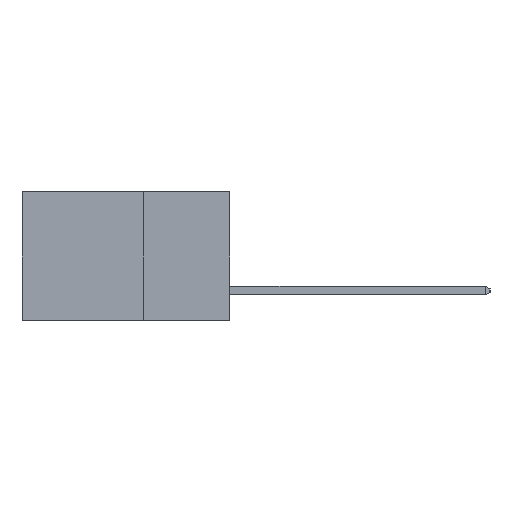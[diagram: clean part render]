
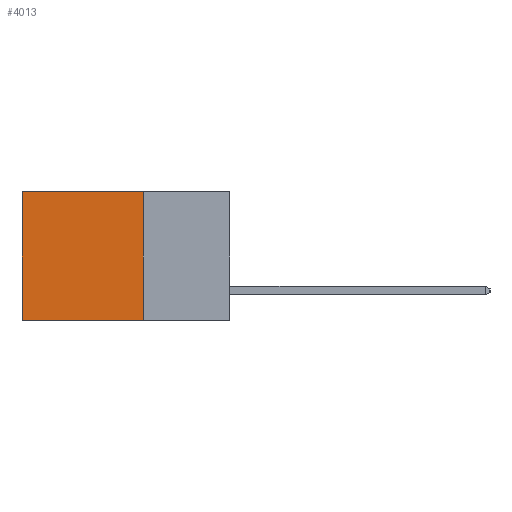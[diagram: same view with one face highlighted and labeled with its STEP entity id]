
A CAD part, left-side view. The second image highlights one B-rep face of the part: STEP entity #4013.
In plain terms, the highlighted planar face has unit normal (-1, 0, 0).
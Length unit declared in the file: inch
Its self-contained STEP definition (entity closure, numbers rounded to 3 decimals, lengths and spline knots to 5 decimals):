
#150 = LINE ( 'NONE', #4947, #2420 ) ;
#373 = EDGE_LOOP ( 'NONE', ( #7798, #1128, #7239, #2101 ) ) ;
#575 = FACE_OUTER_BOUND ( 'NONE', #373, .T. ) ;
#914 = EDGE_CURVE ( 'NONE', #4407, #2104, #3662, .T. ) ;
#1128 = ORIENTED_EDGE ( 'NONE', *, *, #2085, .F. ) ;
#1239 = EDGE_CURVE ( 'NONE', #2104, #10330, #10528, .T. ) ;
#2085 = EDGE_CURVE ( 'NONE', #5070, #10330, #150, .T. ) ;
#2101 = ORIENTED_EDGE ( 'NONE', *, *, #914, .T. ) ;
#2104 = VERTEX_POINT ( 'NONE', #4749 ) ;
#2420 = VECTOR ( 'NONE', #4946, 39.37008 ) ;
#2771 = EDGE_CURVE ( 'NONE', #4407, #5070, #9111, .T. ) ;
#2784 = CARTESIAN_POINT ( 'NONE',  ( 0.2615, 0.25, -0.37 ) ) ;
#3662 = LINE ( 'NONE', #4537, #5960 ) ;
#4013 = ADVANCED_FACE ( 'NONE', ( #575 ), #8514, .F. ) ;
#4407 = VERTEX_POINT ( 'NONE', #6549 ) ;
#4537 = CARTESIAN_POINT ( 'NONE',  ( 0.2615, 0.25, 0. ) ) ;
#4661 = DIRECTION ( 'NONE',  ( 0., 1., 0. ) ) ;
#4749 = CARTESIAN_POINT ( 'NONE',  ( 0.2615, 0.6, 0. ) ) ;
#4946 = DIRECTION ( 'NONE',  ( 0., 1., 0. ) ) ;
#4947 = CARTESIAN_POINT ( 'NONE',  ( 0.2615, 0.25, -0.37 ) ) ;
#5070 = VERTEX_POINT ( 'NONE', #2784 ) ;
#5813 = VECTOR ( 'NONE', #10361, 39.37008 ) ;
#5960 = VECTOR ( 'NONE', #4661, 39.37008 ) ;
#6549 = CARTESIAN_POINT ( 'NONE',  ( 0.2615, 0.25, 0. ) ) ;
#7169 = CARTESIAN_POINT ( 'NONE',  ( 0.2615, 0.6, -0.37 ) ) ;
#7239 = ORIENTED_EDGE ( 'NONE', *, *, #2771, .F. ) ;
#7798 = ORIENTED_EDGE ( 'NONE', *, *, #1239, .T. ) ;
#8469 = DIRECTION ( 'NONE',  ( 0., 0., -1. ) ) ;
#8479 = DIRECTION ( 'NONE',  ( 1., 0., 0. ) ) ;
#8505 = CARTESIAN_POINT ( 'NONE',  ( 0.2615, 0.25, -0.37 ) ) ;
#8514 = PLANE ( 'NONE',  #8553 ) ;
#8553 = AXIS2_PLACEMENT_3D ( 'NONE', #8505, #8479, #8469 ) ;
#9111 = LINE ( 'NONE', #9822, #9361 ) ;
#9361 = VECTOR ( 'NONE', #9728, 39.37008 ) ;
#9728 = DIRECTION ( 'NONE',  ( 0., 0., -1. ) ) ;
#9822 = CARTESIAN_POINT ( 'NONE',  ( 0.2615, 0.25, -0.37 ) ) ;
#10330 = VERTEX_POINT ( 'NONE', #7169 ) ;
#10361 = DIRECTION ( 'NONE',  ( 0., 0., -1. ) ) ;
#10389 = CARTESIAN_POINT ( 'NONE',  ( 0.2615, 0.6, -0.37 ) ) ;
#10528 = LINE ( 'NONE', #10389, #5813 ) ;
